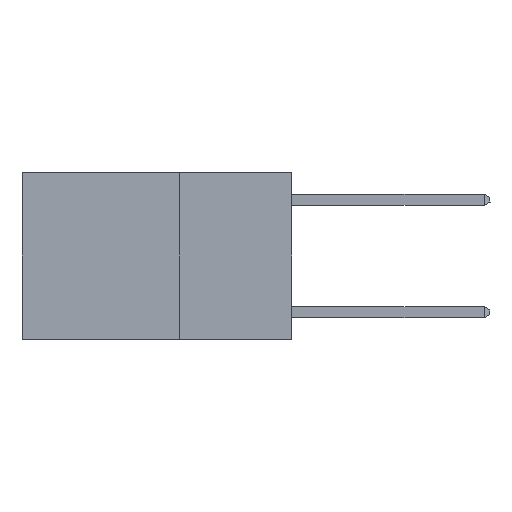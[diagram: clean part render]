
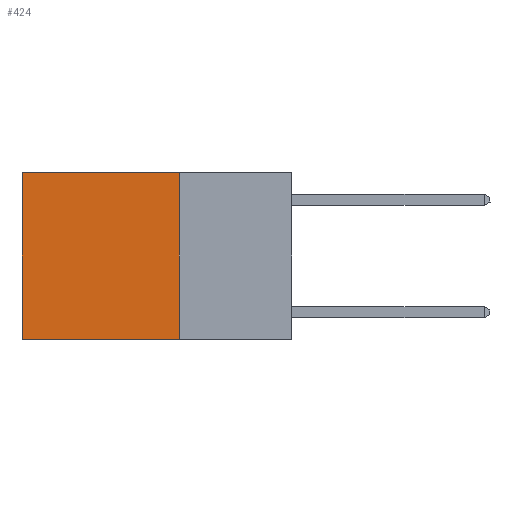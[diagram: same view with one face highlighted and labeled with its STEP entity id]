
A CAD part, left-side view. The second image highlights one B-rep face of the part: STEP entity #424.
In plain terms, the highlighted planar face has unit normal (-1, 0, 0).
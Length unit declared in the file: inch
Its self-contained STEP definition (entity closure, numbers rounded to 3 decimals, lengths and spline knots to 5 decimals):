
#424 = ADVANCED_FACE ( 'NONE', ( #920 ), #9515, .F. ) ;
#920 = FACE_OUTER_BOUND ( 'NONE', #8487, .T. ) ;
#1327 = EDGE_CURVE ( 'NONE', #4720, #4049, #2272, .T. ) ;
#1524 = CARTESIAN_POINT ( 'NONE',  ( 0.2625, 0.25, -0.37 ) ) ;
#1573 = DIRECTION ( 'NONE',  ( 0., 0., -1. ) ) ;
#1677 = CARTESIAN_POINT ( 'NONE',  ( 0.2625, 0.6, -0.37 ) ) ;
#1932 = ORIENTED_EDGE ( 'NONE', *, *, #3441, .T. ) ;
#2233 = ORIENTED_EDGE ( 'NONE', *, *, #7784, .F. ) ;
#2272 = LINE ( 'NONE', #11532, #11044 ) ;
#2302 = LINE ( 'NONE', #7501, #11317 ) ;
#2988 = VERTEX_POINT ( 'NONE', #1677 ) ;
#3441 = EDGE_CURVE ( 'NONE', #4049, #2988, #6646, .T. ) ;
#3768 = CARTESIAN_POINT ( 'NONE',  ( 0.2625, 0.25, -0.37 ) ) ;
#3956 = VERTEX_POINT ( 'NONE', #1524 ) ;
#4049 = VERTEX_POINT ( 'NONE', #6332 ) ;
#4401 = CARTESIAN_POINT ( 'NONE',  ( 0.2625, 0.6, 0. ) ) ;
#4646 = DIRECTION ( 'NONE',  ( 0., 1., 0. ) ) ;
#4720 = VERTEX_POINT ( 'NONE', #7935 ) ;
#5141 = DIRECTION ( 'NONE',  ( 0., 0., -1. ) ) ;
#5218 = EDGE_CURVE ( 'NONE', #3956, #2988, #9376, .T. ) ;
#6332 = CARTESIAN_POINT ( 'NONE',  ( 0.2625, 0.6, 0. ) ) ;
#6646 = LINE ( 'NONE', #4401, #11115 ) ;
#6700 = AXIS2_PLACEMENT_3D ( 'NONE', #7824, #10320, #5141 ) ;
#7097 = VECTOR ( 'NONE', #4646, 39.37008 ) ;
#7104 = ORIENTED_EDGE ( 'NONE', *, *, #1327, .T. ) ;
#7501 = CARTESIAN_POINT ( 'NONE',  ( 0.2625, 0.25, 0. ) ) ;
#7784 = EDGE_CURVE ( 'NONE', #4720, #3956, #2302, .T. ) ;
#7824 = CARTESIAN_POINT ( 'NONE',  ( 0.2625, 0.25, 0. ) ) ;
#7935 = CARTESIAN_POINT ( 'NONE',  ( 0.2625, 0.25, 0. ) ) ;
#8487 = EDGE_LOOP ( 'NONE', ( #1932, #11262, #2233, #7104 ) ) ;
#9376 = LINE ( 'NONE', #3768, #7097 ) ;
#9515 = PLANE ( 'NONE',  #6700 ) ;
#9915 = DIRECTION ( 'NONE',  ( 0., 1., 0. ) ) ;
#10008 = DIRECTION ( 'NONE',  ( 0., 0., -1. ) ) ;
#10320 = DIRECTION ( 'NONE',  ( 1., 0., 0. ) ) ;
#11044 = VECTOR ( 'NONE', #9915, 39.37008 ) ;
#11115 = VECTOR ( 'NONE', #1573, 39.37008 ) ;
#11262 = ORIENTED_EDGE ( 'NONE', *, *, #5218, .F. ) ;
#11317 = VECTOR ( 'NONE', #10008, 39.37008 ) ;
#11532 = CARTESIAN_POINT ( 'NONE',  ( 0.2625, 0.25, 0. ) ) ;
